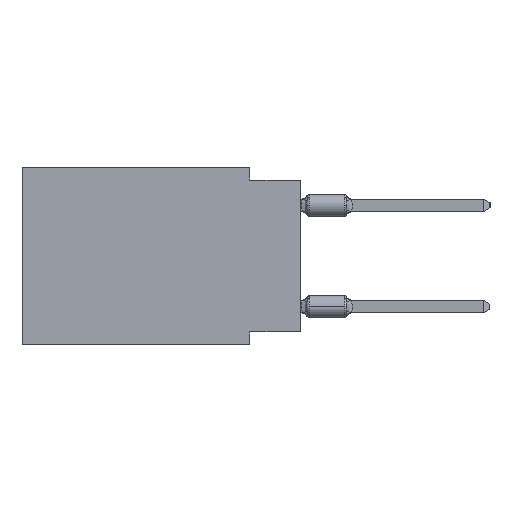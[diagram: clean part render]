
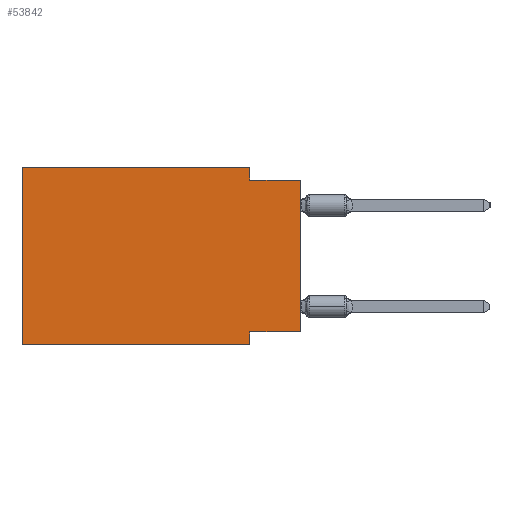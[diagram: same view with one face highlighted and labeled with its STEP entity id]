
A CAD part, left-side view. The second image highlights one B-rep face of the part: STEP entity #53842.
In plain terms, the highlighted planar face has unit normal (-1, 0, 0).
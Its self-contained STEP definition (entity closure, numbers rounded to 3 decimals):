
#444 = CARTESIAN_POINT ( 'NONE',  ( 0., 2.54, -0.635 ) ) ;
#1149 = EDGE_CURVE ( 'NONE', #17658, #35766, #24414, .T. ) ;
#2489 = VERTEX_POINT ( 'NONE', #12638 ) ;
#3602 = EDGE_CURVE ( 'NONE', #28176, #2489, #37137, .T. ) ;
#3700 = CARTESIAN_POINT ( 'NONE',  ( 0., 0., -8.255 ) ) ;
#3933 = CARTESIAN_POINT ( 'NONE',  ( 0., 13.97, -8.89 ) ) ;
#5492 = VECTOR ( 'NONE', #35453, 1000. ) ;
#6243 = EDGE_CURVE ( 'NONE', #21650, #2489, #8490, .T. ) ;
#6783 = ORIENTED_EDGE ( 'NONE', *, *, #3602, .F. ) ;
#7094 = DIRECTION ( 'NONE',  ( 0., 1., 0. ) ) ;
#8490 = LINE ( 'NONE', #3933, #44856 ) ;
#9359 = CARTESIAN_POINT ( 'NONE',  ( 0., 2.54, 0. ) ) ;
#10640 = FACE_OUTER_BOUND ( 'NONE', #43172, .T. ) ;
#10865 = VECTOR ( 'NONE', #38407, 1000. ) ;
#12638 = CARTESIAN_POINT ( 'NONE',  ( 0., 2.54, -8.89 ) ) ;
#12731 = CARTESIAN_POINT ( 'NONE',  ( 0., 0., 0. ) ) ;
#12893 = CARTESIAN_POINT ( 'NONE',  ( 0., 13.97, -8.89 ) ) ;
#13117 = EDGE_CURVE ( 'NONE', #55967, #28176, #45490, .T. ) ;
#13890 = EDGE_CURVE ( 'NONE', #35766, #30255, #20031, .T. ) ;
#14279 = CARTESIAN_POINT ( 'NONE',  ( 0., 2.54, 0. ) ) ;
#14708 = VECTOR ( 'NONE', #15817, 1000. ) ;
#15817 = DIRECTION ( 'NONE',  ( 0., 0., -1. ) ) ;
#17658 = VERTEX_POINT ( 'NONE', #9359 ) ;
#18336 = AXIS2_PLACEMENT_3D ( 'NONE', #45323, #41354, #40779 ) ;
#18409 = CARTESIAN_POINT ( 'NONE',  ( 0., 13.97, 0. ) ) ;
#18536 = VECTOR ( 'NONE', #7094, 1000. ) ;
#19171 = PLANE ( 'NONE',  #18336 ) ;
#20031 = LINE ( 'NONE', #24284, #40340 ) ;
#20901 = EDGE_CURVE ( 'NONE', #21650, #53635, #27485, .T. ) ;
#21650 = VERTEX_POINT ( 'NONE', #12893 ) ;
#24284 = CARTESIAN_POINT ( 'NONE',  ( 0., 0., -0.635 ) ) ;
#24414 = LINE ( 'NONE', #14279, #33542 ) ;
#24990 = EDGE_CURVE ( 'NONE', #55967, #30255, #38608, .T. ) ;
#25390 = CARTESIAN_POINT ( 'NONE',  ( 0., 0., -0.635 ) ) ;
#25751 = ORIENTED_EDGE ( 'NONE', *, *, #13890, .F. ) ;
#27485 = LINE ( 'NONE', #18409, #5492 ) ;
#27844 = ORIENTED_EDGE ( 'NONE', *, *, #20901, .F. ) ;
#28158 = CARTESIAN_POINT ( 'NONE',  ( 0., 2.54, -8.255 ) ) ;
#28176 = VERTEX_POINT ( 'NONE', #28158 ) ;
#29855 = LINE ( 'NONE', #38954, #10865 ) ;
#30255 = VERTEX_POINT ( 'NONE', #25390 ) ;
#33542 = VECTOR ( 'NONE', #44405, 1000. ) ;
#35453 = DIRECTION ( 'NONE',  ( 0., 0., 1. ) ) ;
#35766 = VERTEX_POINT ( 'NONE', #444 ) ;
#36430 = ORIENTED_EDGE ( 'NONE', *, *, #13117, .F. ) ;
#36523 = ORIENTED_EDGE ( 'NONE', *, *, #1149, .F. ) ;
#37137 = LINE ( 'NONE', #41968, #14708 ) ;
#38407 = DIRECTION ( 'NONE',  ( 0., -1., 0. ) ) ;
#38608 = LINE ( 'NONE', #12731, #41983 ) ;
#38954 = CARTESIAN_POINT ( 'NONE',  ( 0., 13.97, 0. ) ) ;
#40340 = VECTOR ( 'NONE', #45625, 1000. ) ;
#40779 = DIRECTION ( 'NONE',  ( 0., 0., -1. ) ) ;
#41354 = DIRECTION ( 'NONE',  ( 1., 0., 0. ) ) ;
#41968 = CARTESIAN_POINT ( 'NONE',  ( 0., 2.54, -8.89 ) ) ;
#41983 = VECTOR ( 'NONE', #42596, 1000. ) ;
#42596 = DIRECTION ( 'NONE',  ( 0., 0., 1. ) ) ;
#42627 = DIRECTION ( 'NONE',  ( 0., -1., 0. ) ) ;
#43172 = EDGE_LOOP ( 'NONE', ( #47345, #25751, #36523, #48348, #27844, #44294, #6783, #36430 ) ) ;
#44294 = ORIENTED_EDGE ( 'NONE', *, *, #6243, .T. ) ;
#44405 = DIRECTION ( 'NONE',  ( 0., 0., -1. ) ) ;
#44856 = VECTOR ( 'NONE', #42627, 1000. ) ;
#45323 = CARTESIAN_POINT ( 'NONE',  ( 0., 13.97, 0. ) ) ;
#45490 = LINE ( 'NONE', #54020, #18536 ) ;
#45625 = DIRECTION ( 'NONE',  ( 0., -1., 0. ) ) ;
#47345 = ORIENTED_EDGE ( 'NONE', *, *, #24990, .T. ) ;
#47611 = CARTESIAN_POINT ( 'NONE',  ( 0., 13.97, 0. ) ) ;
#48348 = ORIENTED_EDGE ( 'NONE', *, *, #55982, .F. ) ;
#53635 = VERTEX_POINT ( 'NONE', #47611 ) ;
#53842 = ADVANCED_FACE ( 'NONE', ( #10640 ), #19171, .F. ) ;
#54020 = CARTESIAN_POINT ( 'NONE',  ( 0., 0., -8.255 ) ) ;
#55967 = VERTEX_POINT ( 'NONE', #3700 ) ;
#55982 = EDGE_CURVE ( 'NONE', #53635, #17658, #29855, .T. ) ;
